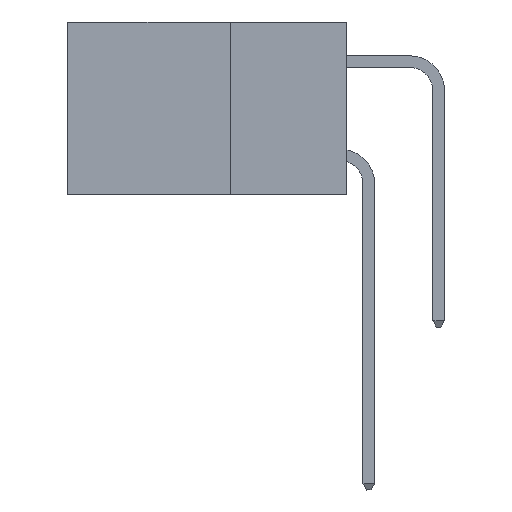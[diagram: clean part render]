
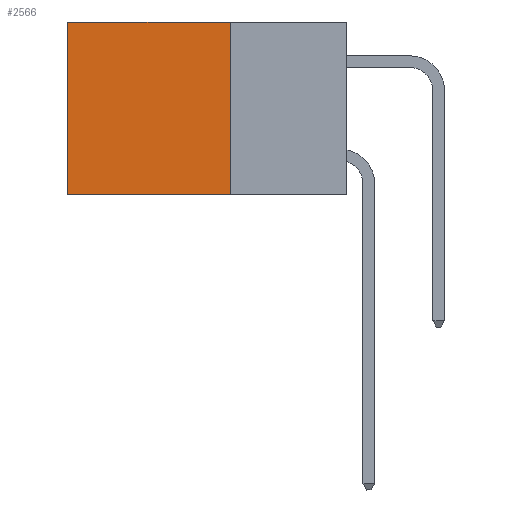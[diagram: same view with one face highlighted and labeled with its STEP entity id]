
A CAD part, left-side view. The second image highlights one B-rep face of the part: STEP entity #2566.
In plain terms, the highlighted planar face has unit normal (-1, 0, 0).
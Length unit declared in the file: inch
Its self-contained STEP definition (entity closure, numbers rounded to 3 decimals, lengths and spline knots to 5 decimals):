
#21 = VECTOR ( 'NONE', #863, 39.37008 ) ;
#22 = VECTOR ( 'NONE', #627, 39.37008 ) ;
#464 = ORIENTED_EDGE ( 'NONE', *, *, #1020, .T. ) ;
#627 = DIRECTION ( 'NONE',  ( 0., 0., -1. ) ) ;
#863 = DIRECTION ( 'NONE',  ( 0., 0., -1. ) ) ;
#1020 = EDGE_CURVE ( 'NONE', #7728, #14787, #2873, .T. ) ;
#1433 = DIRECTION ( 'NONE',  ( 0., 0., -1. ) ) ;
#2273 = CARTESIAN_POINT ( 'NONE',  ( 0.2875, 0.6, -0.37 ) ) ;
#2566 = ADVANCED_FACE ( 'NONE', ( #4956 ), #10782, .F. ) ;
#2779 = DIRECTION ( 'NONE',  ( 0., 1., 0. ) ) ;
#2873 = LINE ( 'NONE', #10015, #8763 ) ;
#3228 = LINE ( 'NONE', #7481, #6372 ) ;
#4956 = FACE_OUTER_BOUND ( 'NONE', #11230, .T. ) ;
#5339 = ORIENTED_EDGE ( 'NONE', *, *, #8132, .F. ) ;
#5819 = VERTEX_POINT ( 'NONE', #9298 ) ;
#5945 = CARTESIAN_POINT ( 'NONE',  ( 0.2875, 0.6, 0. ) ) ;
#6372 = VECTOR ( 'NONE', #2779, 39.37008 ) ;
#7102 = EDGE_CURVE ( 'NONE', #7728, #5819, #9432, .T. ) ;
#7358 = CARTESIAN_POINT ( 'NONE',  ( 0.2875, 0.25, 0. ) ) ;
#7481 = CARTESIAN_POINT ( 'NONE',  ( 0.2875, 0.25, -0.37 ) ) ;
#7728 = VERTEX_POINT ( 'NONE', #14712 ) ;
#7966 = CARTESIAN_POINT ( 'NONE',  ( 0.2875, 0.25, 0. ) ) ;
#8008 = DIRECTION ( 'NONE',  ( 0., 1., 0. ) ) ;
#8132 = EDGE_CURVE ( 'NONE', #5819, #8564, #3228, .T. ) ;
#8523 = DIRECTION ( 'NONE',  ( 1., 0., 0. ) ) ;
#8564 = VERTEX_POINT ( 'NONE', #2273 ) ;
#8743 = ORIENTED_EDGE ( 'NONE', *, *, #13838, .T. ) ;
#8763 = VECTOR ( 'NONE', #8008, 39.37008 ) ;
#9088 = LINE ( 'NONE', #12344, #22 ) ;
#9298 = CARTESIAN_POINT ( 'NONE',  ( 0.2875, 0.25, -0.37 ) ) ;
#9432 = LINE ( 'NONE', #7966, #21 ) ;
#10015 = CARTESIAN_POINT ( 'NONE',  ( 0.2875, 0.25, 0. ) ) ;
#10782 = PLANE ( 'NONE',  #13530 ) ;
#11230 = EDGE_LOOP ( 'NONE', ( #8743, #5339, #14930, #464 ) ) ;
#12344 = CARTESIAN_POINT ( 'NONE',  ( 0.2875, 0.6, 0. ) ) ;
#13530 = AXIS2_PLACEMENT_3D ( 'NONE', #7358, #8523, #1433 ) ;
#13838 = EDGE_CURVE ( 'NONE', #14787, #8564, #9088, .T. ) ;
#14712 = CARTESIAN_POINT ( 'NONE',  ( 0.2875, 0.25, 0. ) ) ;
#14787 = VERTEX_POINT ( 'NONE', #5945 ) ;
#14930 = ORIENTED_EDGE ( 'NONE', *, *, #7102, .F. ) ;
